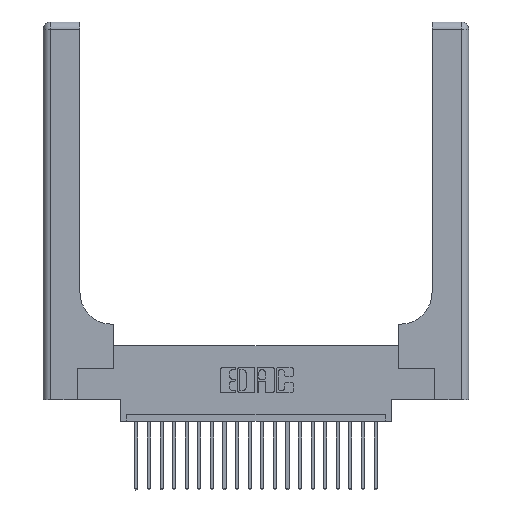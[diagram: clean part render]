
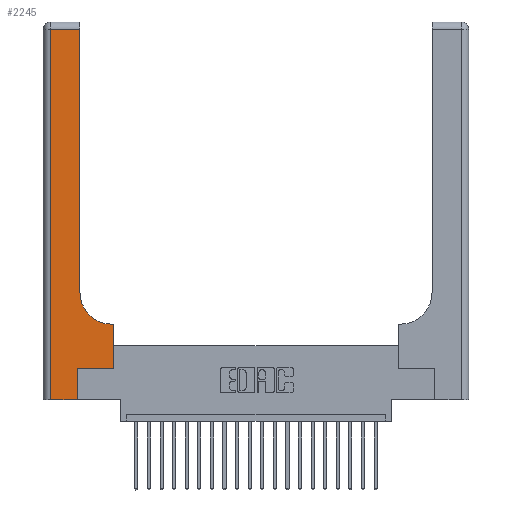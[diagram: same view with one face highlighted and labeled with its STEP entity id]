
A CAD part, top view. The second image highlights one B-rep face of the part: STEP entity #2245.
In plain terms, the highlighted planar face has unit normal (0, 0, 1).
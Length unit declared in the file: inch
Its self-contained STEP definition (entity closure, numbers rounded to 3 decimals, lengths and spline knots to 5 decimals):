
#244 = VECTOR ( 'NONE', #2317, 39.37008 ) ;
#1301 = DIRECTION ( 'NONE',  ( 0., 1., 0. ) ) ;
#2245 = ADVANCED_FACE ( 'NONE', ( #14107 ), #19564, .F. ) ;
#2317 = DIRECTION ( 'NONE',  ( 0., 1., 0. ) ) ;
#2440 = VERTEX_POINT ( 'NONE', #19076 ) ;
#2645 = DIRECTION ( 'NONE',  ( 1., 0., 0. ) ) ;
#3559 = VERTEX_POINT ( 'NONE', #11562 ) ;
#3677 = AXIS2_PLACEMENT_3D ( 'NONE', #17057, #19093, #2645 ) ;
#3815 = CARTESIAN_POINT ( 'NONE',  ( 0.269, 0., 0.37 ) ) ;
#3826 = EDGE_CURVE ( 'NONE', #17354, #15684, #13769, .T. ) ;
#4228 = EDGE_CURVE ( 'NONE', #16145, #17354, #17147, .T. ) ;
#4522 = VERTEX_POINT ( 'NONE', #5855 ) ;
#4946 = VECTOR ( 'NONE', #9008, 39.37008 ) ;
#5139 = LINE ( 'NONE', #21354, #12765 ) ;
#5212 = CARTESIAN_POINT ( 'NONE',  ( 0., 0., 0.37 ) ) ;
#5305 = VECTOR ( 'NONE', #19716, 39.37008 ) ;
#5408 = ORIENTED_EDGE ( 'NONE', *, *, #7439, .T. ) ;
#5482 = ORIENTED_EDGE ( 'NONE', *, *, #16373, .T. ) ;
#5491 = VECTOR ( 'NONE', #11006, 39.37008 ) ;
#5579 = LINE ( 'NONE', #12111, #18208 ) ;
#5849 = ORIENTED_EDGE ( 'NONE', *, *, #19604, .T. ) ;
#5855 = CARTESIAN_POINT ( 'NONE',  ( 0.269, 0.25, 0.37 ) ) ;
#6008 = VECTOR ( 'NONE', #8417, 39.37008 ) ;
#6178 = CARTESIAN_POINT ( 'NONE',  ( 0.5585, 0.25, 0.37 ) ) ;
#7439 = EDGE_CURVE ( 'NONE', #2440, #22982, #15704, .T. ) ;
#7587 = CARTESIAN_POINT ( 'NONE',  ( 0.2915, 2.94, 0.37 ) ) ;
#8417 = DIRECTION ( 'NONE',  ( -1., 0., 0. ) ) ;
#9008 = DIRECTION ( 'NONE',  ( 0., -1., 0. ) ) ;
#9387 = EDGE_CURVE ( 'NONE', #4522, #17287, #15068, .T. ) ;
#10099 = DIRECTION ( 'NONE',  ( 0., 1., 0. ) ) ;
#10241 = CARTESIAN_POINT ( 'NONE',  ( 0.269, 0., 0.37 ) ) ;
#10611 = CARTESIAN_POINT ( 'NONE',  ( 0., 3., 0.37 ) ) ;
#11006 = DIRECTION ( 'NONE',  ( 1., 0., 0. ) ) ;
#11080 = LINE ( 'NONE', #22618, #6008 ) ;
#11386 = CARTESIAN_POINT ( 'NONE',  ( 0.2915, 0.85, 0.37 ) ) ;
#11562 = CARTESIAN_POINT ( 'NONE',  ( 0.06, 2.94, 0.37 ) ) ;
#12111 = CARTESIAN_POINT ( 'NONE',  ( 0.5585, 0.25, 0.37 ) ) ;
#12395 = CARTESIAN_POINT ( 'NONE',  ( 0.5415, 0.6, 0.37 ) ) ;
#12693 = CARTESIAN_POINT ( 'NONE',  ( 0.269, 0.25, 0.37 ) ) ;
#12765 = VECTOR ( 'NONE', #14481, 39.37008 ) ;
#13006 = VERTEX_POINT ( 'NONE', #16027 ) ;
#13769 = LINE ( 'NONE', #18710, #244 ) ;
#14107 = FACE_OUTER_BOUND ( 'NONE', #21800, .T. ) ;
#14199 = DIRECTION ( 'NONE',  ( 0., 0., -1. ) ) ;
#14481 = DIRECTION ( 'NONE',  ( -1., 0., 0. ) ) ;
#15068 = LINE ( 'NONE', #12693, #5491 ) ;
#15470 = EDGE_CURVE ( 'NONE', #17287, #13006, #5579, .T. ) ;
#15684 = VERTEX_POINT ( 'NONE', #7587 ) ;
#15704 = LINE ( 'NONE', #5212, #5305 ) ;
#16019 = DIRECTION ( 'NONE',  ( -1., 0., 0. ) ) ;
#16027 = CARTESIAN_POINT ( 'NONE',  ( 0.5585, 0.6, 0.37 ) ) ;
#16145 = VERTEX_POINT ( 'NONE', #12395 ) ;
#16373 = EDGE_CURVE ( 'NONE', #3559, #2440, #17914, .T. ) ;
#16800 = ORIENTED_EDGE ( 'NONE', *, *, #4228, .T. ) ;
#17057 = CARTESIAN_POINT ( 'NONE',  ( 0.5415, 0.85, 0.37 ) ) ;
#17147 = CIRCLE ( 'NONE', #3677, 0.25 ) ;
#17287 = VERTEX_POINT ( 'NONE', #6178 ) ;
#17354 = VERTEX_POINT ( 'NONE', #11386 ) ;
#17866 = AXIS2_PLACEMENT_3D ( 'NONE', #10611, #14199, #16019 ) ;
#17914 = LINE ( 'NONE', #19712, #4946 ) ;
#18208 = VECTOR ( 'NONE', #1301, 39.37008 ) ;
#18659 = ORIENTED_EDGE ( 'NONE', *, *, #9387, .T. ) ;
#18710 = CARTESIAN_POINT ( 'NONE',  ( 0.2915, 3., 0.37 ) ) ;
#19061 = ORIENTED_EDGE ( 'NONE', *, *, #19194, .T. ) ;
#19076 = CARTESIAN_POINT ( 'NONE',  ( 0.06, 0., 0.37 ) ) ;
#19093 = DIRECTION ( 'NONE',  ( 0., 0., -1. ) ) ;
#19194 = EDGE_CURVE ( 'NONE', #15684, #3559, #5139, .T. ) ;
#19564 = PLANE ( 'NONE',  #17866 ) ;
#19604 = EDGE_CURVE ( 'NONE', #13006, #16145, #11080, .T. ) ;
#19671 = EDGE_CURVE ( 'NONE', #22982, #4522, #21793, .T. ) ;
#19712 = CARTESIAN_POINT ( 'NONE',  ( 0.06, 3., 0.37 ) ) ;
#19716 = DIRECTION ( 'NONE',  ( 1., 0., 0. ) ) ;
#20099 = ORIENTED_EDGE ( 'NONE', *, *, #15470, .T. ) ;
#21215 = VECTOR ( 'NONE', #10099, 39.37008 ) ;
#21323 = ORIENTED_EDGE ( 'NONE', *, *, #19671, .T. ) ;
#21354 = CARTESIAN_POINT ( 'NONE',  ( 0., 2.94, 0.37 ) ) ;
#21702 = ORIENTED_EDGE ( 'NONE', *, *, #3826, .T. ) ;
#21793 = LINE ( 'NONE', #10241, #21215 ) ;
#21800 = EDGE_LOOP ( 'NONE', ( #21702, #19061, #5482, #5408, #21323, #18659, #20099, #5849, #16800 ) ) ;
#22618 = CARTESIAN_POINT ( 'NONE',  ( 0.2915, 0.6, 0.37 ) ) ;
#22982 = VERTEX_POINT ( 'NONE', #3815 ) ;
